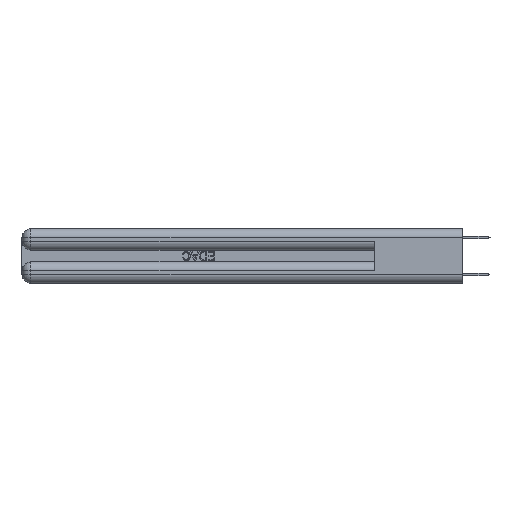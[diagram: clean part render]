
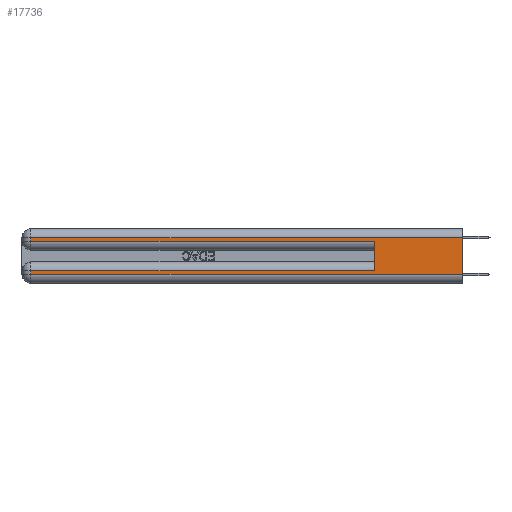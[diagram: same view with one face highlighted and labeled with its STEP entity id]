
A CAD part, left-side view. The second image highlights one B-rep face of the part: STEP entity #17736.
In plain terms, the highlighted planar face has unit normal (-1, 0, 0).
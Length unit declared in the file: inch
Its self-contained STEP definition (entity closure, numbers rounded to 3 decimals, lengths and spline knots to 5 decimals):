
#635 = CARTESIAN_POINT ( 'NONE',  ( 0., 2.94, 0.085 ) ) ;
#796 = CARTESIAN_POINT ( 'NONE',  ( 0., 2.94, 0.31 ) ) ;
#1302 = LINE ( 'NONE', #31553, #16681 ) ;
#1666 = VECTOR ( 'NONE', #27941, 39.37008 ) ;
#2134 = VERTEX_POINT ( 'NONE', #25321 ) ;
#2237 = CARTESIAN_POINT ( 'NONE',  ( 0., 0., 0.285 ) ) ;
#2519 = DIRECTION ( 'NONE',  ( 1., 0., 0. ) ) ;
#2750 = CARTESIAN_POINT ( 'NONE',  ( 0., 0., 0.06 ) ) ;
#2901 = CARTESIAN_POINT ( 'NONE',  ( 0., 0., 0.37 ) ) ;
#5742 = DIRECTION ( 'NONE',  ( 0., 0., 1. ) ) ;
#6747 = CARTESIAN_POINT ( 'NONE',  ( 0., 0.6, 0.085 ) ) ;
#6783 = LINE ( 'NONE', #13900, #34088 ) ;
#6897 = EDGE_CURVE ( 'NONE', #18812, #10206, #23120, .T. ) ;
#7274 = CARTESIAN_POINT ( 'NONE',  ( 0., 2.94, 0.285 ) ) ;
#7583 = FACE_OUTER_BOUND ( 'NONE', #27670, .T. ) ;
#8275 = ORIENTED_EDGE ( 'NONE', *, *, #28927, .T. ) ;
#8712 = VERTEX_POINT ( 'NONE', #20045 ) ;
#9389 = VERTEX_POINT ( 'NONE', #6747 ) ;
#9929 = VERTEX_POINT ( 'NONE', #12673 ) ;
#10206 = VERTEX_POINT ( 'NONE', #7274 ) ;
#10787 = DIRECTION ( 'NONE',  ( 0., 0., -1. ) ) ;
#12517 = VECTOR ( 'NONE', #12629, 39.37008 ) ;
#12629 = DIRECTION ( 'NONE',  ( 0., 0., -1. ) ) ;
#12673 = CARTESIAN_POINT ( 'NONE',  ( 0., 0.6, 0.285 ) ) ;
#13272 = LINE ( 'NONE', #2750, #14130 ) ;
#13387 = VECTOR ( 'NONE', #18832, 39.37008 ) ;
#13900 = CARTESIAN_POINT ( 'NONE',  ( 0., 0.6, 0.145 ) ) ;
#14130 = VECTOR ( 'NONE', #24557, 39.37008 ) ;
#16681 = VECTOR ( 'NONE', #17841, 39.37008 ) ;
#16783 = ORIENTED_EDGE ( 'NONE', *, *, #26874, .F. ) ;
#17454 = LINE ( 'NONE', #19720, #1666 ) ;
#17736 = ADVANCED_FACE ( 'NONE', ( #7583 ), #35199, .F. ) ;
#17841 = DIRECTION ( 'NONE',  ( 0., 1., 0. ) ) ;
#18057 = LINE ( 'NONE', #2237, #13387 ) ;
#18071 = VECTOR ( 'NONE', #24824, 39.37008 ) ;
#18227 = CARTESIAN_POINT ( 'NONE',  ( 0., 0., 0.06 ) ) ;
#18812 = VERTEX_POINT ( 'NONE', #796 ) ;
#18832 = DIRECTION ( 'NONE',  ( 0., -1., 0. ) ) ;
#18850 = EDGE_CURVE ( 'NONE', #19586, #2134, #23704, .T. ) ;
#19341 = EDGE_CURVE ( 'NONE', #10206, #9929, #18057, .T. ) ;
#19586 = VERTEX_POINT ( 'NONE', #635 ) ;
#19720 = CARTESIAN_POINT ( 'NONE',  ( 0., 0., 0.085 ) ) ;
#20045 = CARTESIAN_POINT ( 'NONE',  ( 0., 0., 0.31 ) ) ;
#21861 = LINE ( 'NONE', #2901, #18071 ) ;
#22191 = AXIS2_PLACEMENT_3D ( 'NONE', #24199, #2519, #10787 ) ;
#22752 = CARTESIAN_POINT ( 'NONE',  ( 0., 2.94, 0.37 ) ) ;
#23120 = LINE ( 'NONE', #23438, #12517 ) ;
#23165 = EDGE_CURVE ( 'NONE', #8712, #18812, #1302, .T. ) ;
#23438 = CARTESIAN_POINT ( 'NONE',  ( 0., 2.94, 0.37 ) ) ;
#23704 = LINE ( 'NONE', #22752, #25419 ) ;
#24199 = CARTESIAN_POINT ( 'NONE',  ( 0., 0., 0.37 ) ) ;
#24392 = ORIENTED_EDGE ( 'NONE', *, *, #19341, .T. ) ;
#24413 = ORIENTED_EDGE ( 'NONE', *, *, #6897, .T. ) ;
#24557 = DIRECTION ( 'NONE',  ( 0., -1., 0. ) ) ;
#24824 = DIRECTION ( 'NONE',  ( 0., 0., -1. ) ) ;
#25321 = CARTESIAN_POINT ( 'NONE',  ( 0., 2.94, 0.06 ) ) ;
#25419 = VECTOR ( 'NONE', #30555, 39.37008 ) ;
#26874 = EDGE_CURVE ( 'NONE', #8712, #29920, #21861, .T. ) ;
#27305 = ORIENTED_EDGE ( 'NONE', *, *, #23165, .T. ) ;
#27670 = EDGE_LOOP ( 'NONE', ( #16783, #27305, #24413, #24392, #34697, #34122, #28633, #8275 ) ) ;
#27941 = DIRECTION ( 'NONE',  ( 0., 1., 0. ) ) ;
#28633 = ORIENTED_EDGE ( 'NONE', *, *, #18850, .T. ) ;
#28927 = EDGE_CURVE ( 'NONE', #2134, #29920, #13272, .T. ) ;
#29920 = VERTEX_POINT ( 'NONE', #18227 ) ;
#30555 = DIRECTION ( 'NONE',  ( 0., 0., -1. ) ) ;
#31553 = CARTESIAN_POINT ( 'NONE',  ( 0., 0., 0.31 ) ) ;
#34042 = EDGE_CURVE ( 'NONE', #9389, #9929, #6783, .T. ) ;
#34088 = VECTOR ( 'NONE', #5742, 39.37008 ) ;
#34122 = ORIENTED_EDGE ( 'NONE', *, *, #34184, .T. ) ;
#34184 = EDGE_CURVE ( 'NONE', #9389, #19586, #17454, .T. ) ;
#34697 = ORIENTED_EDGE ( 'NONE', *, *, #34042, .F. ) ;
#35199 = PLANE ( 'NONE',  #22191 ) ;
